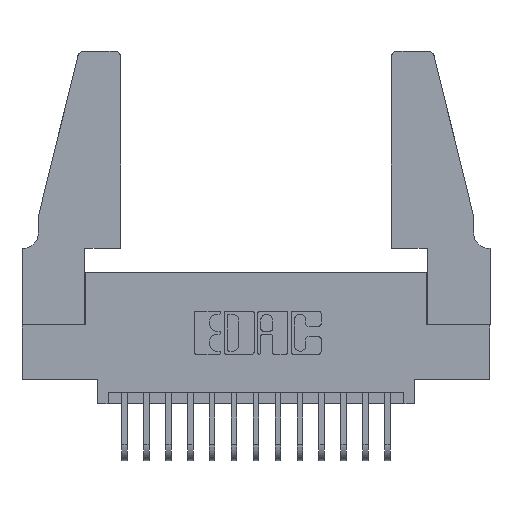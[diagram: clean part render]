
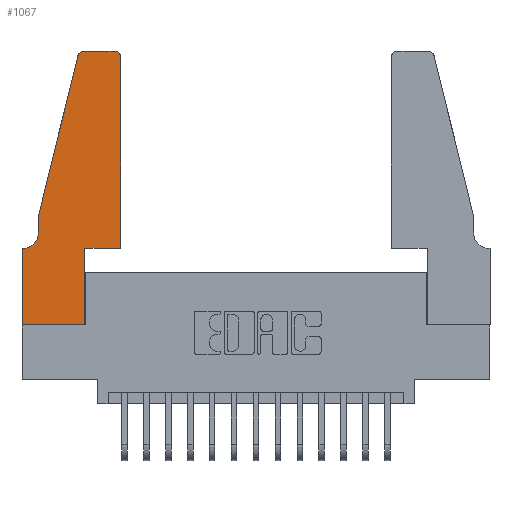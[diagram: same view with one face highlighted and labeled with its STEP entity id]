
A CAD part, top view. The second image highlights one B-rep face of the part: STEP entity #1067.
In plain terms, the highlighted planar face has unit normal (0, 0, 1).
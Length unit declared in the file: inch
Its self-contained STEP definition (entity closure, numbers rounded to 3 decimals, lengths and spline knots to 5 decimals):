
#65 = CARTESIAN_POINT ( 'NONE',  ( 0.0755, 0.42, 0.37 ) ) ;
#125 = EDGE_CURVE ( 'NONE', #2252, #11261, #17638, .T. ) ;
#513 = VERTEX_POINT ( 'NONE', #16929 ) ;
#578 = CARTESIAN_POINT ( 'NONE',  ( 0.4205, 1.25, 0.37 ) ) ;
#634 = AXIS2_PLACEMENT_3D ( 'NONE', #13334, #13268, #6420 ) ;
#637 = CARTESIAN_POINT ( 'NONE',  ( 0.0755, 0.5, 0.37 ) ) ;
#808 = VECTOR ( 'NONE', #11816, 39.37008 ) ;
#824 = LINE ( 'NONE', #6485, #16136 ) ;
#983 = DIRECTION ( 'NONE',  ( -1., 0., 0. ) ) ;
#1049 = FACE_OUTER_BOUND ( 'NONE', #17649, .T. ) ;
#1067 = ADVANCED_FACE ( 'NONE', ( #1049 ), #9913, .T. ) ;
#1149 = VERTEX_POINT ( 'NONE', #11786 ) ;
#1755 = VECTOR ( 'NONE', #6191, 39.37008 ) ;
#1873 = VECTOR ( 'NONE', #3995, 39.37008 ) ;
#1917 = EDGE_CURVE ( 'NONE', #16193, #4725, #12198, .T. ) ;
#2159 = ORIENTED_EDGE ( 'NONE', *, *, #4763, .T. ) ;
#2252 = VERTEX_POINT ( 'NONE', #17783 ) ;
#2263 = VERTEX_POINT ( 'NONE', #15081 ) ;
#2290 = CARTESIAN_POINT ( 'NONE',  ( 0.4505, 0.35, 0.37 ) ) ;
#2453 = VECTOR ( 'NONE', #6379, 39.37008 ) ;
#2570 = EDGE_CURVE ( 'NONE', #1149, #5640, #5826, .T. ) ;
#2689 = DIRECTION ( 'NONE',  ( -1., 0., 0. ) ) ;
#2942 = CARTESIAN_POINT ( 'NONE',  ( 0.4505, 1.22, 0.37 ) ) ;
#3301 = EDGE_CURVE ( 'NONE', #8557, #16193, #14102, .T. ) ;
#3618 = CARTESIAN_POINT ( 'NONE',  ( 0.0055, 0.42, 0.37 ) ) ;
#3658 = LINE ( 'NONE', #13095, #808 ) ;
#3781 = CARTESIAN_POINT ( 'NONE',  ( 0.2605, 1.25, 0.37 ) ) ;
#3995 = DIRECTION ( 'NONE',  ( 0., -1., 0. ) ) ;
#4294 = CARTESIAN_POINT ( 'NONE',  ( 0.4505, 0.35, 0.37 ) ) ;
#4725 = VERTEX_POINT ( 'NONE', #13621 ) ;
#4763 = EDGE_CURVE ( 'NONE', #13131, #1149, #14259, .T. ) ;
#4958 = ORIENTED_EDGE ( 'NONE', *, *, #9117, .T. ) ;
#5321 = AXIS2_PLACEMENT_3D ( 'NONE', #6954, #12606, #12714 ) ;
#5372 = CARTESIAN_POINT ( 'NONE',  ( 0., 0., 0.37 ) ) ;
#5410 = DIRECTION ( 'NONE',  ( 1., 0., 0. ) ) ;
#5640 = VERTEX_POINT ( 'NONE', #15334 ) ;
#5826 = LINE ( 'NONE', #18016, #9329 ) ;
#6191 = DIRECTION ( 'NONE',  ( 1., 0., 0. ) ) ;
#6379 = DIRECTION ( 'NONE',  ( 0., 1., 0. ) ) ;
#6420 = DIRECTION ( 'NONE',  ( 1., 0., 0. ) ) ;
#6443 = EDGE_CURVE ( 'NONE', #4725, #13131, #824, .T. ) ;
#6485 = CARTESIAN_POINT ( 'NONE',  ( 0.0755, 0.35, 0.37 ) ) ;
#6578 = DIRECTION ( 'NONE',  ( -1., 0., 0. ) ) ;
#6681 = EDGE_CURVE ( 'NONE', #2263, #8557, #3658, .T. ) ;
#6808 = LINE ( 'NONE', #3781, #9019 ) ;
#6883 = ORIENTED_EDGE ( 'NONE', *, *, #6443, .T. ) ;
#6954 = CARTESIAN_POINT ( 'NONE',  ( 0., 0.35, 0.37 ) ) ;
#6996 = ORIENTED_EDGE ( 'NONE', *, *, #16022, .T. ) ;
#7057 = AXIS2_PLACEMENT_3D ( 'NONE', #17358, #11962, #12019 ) ;
#7079 = ORIENTED_EDGE ( 'NONE', *, *, #6681, .T. ) ;
#7808 = DIRECTION ( 'NONE',  ( 0., 1., 0. ) ) ;
#7875 = DIRECTION ( 'NONE',  ( 0., 0., -1. ) ) ;
#8315 = ORIENTED_EDGE ( 'NONE', *, *, #10479, .T. ) ;
#8455 = VERTEX_POINT ( 'NONE', #578 ) ;
#8557 = VERTEX_POINT ( 'NONE', #637 ) ;
#9019 = VECTOR ( 'NONE', #983, 39.37008 ) ;
#9117 = EDGE_CURVE ( 'NONE', #513, #2263, #11643, .T. ) ;
#9329 = VECTOR ( 'NONE', #5410, 39.37008 ) ;
#9556 = CARTESIAN_POINT ( 'NONE',  ( 0.0755, 0.5, 0.37 ) ) ;
#9913 = PLANE ( 'NONE',  #5321 ) ;
#10322 = ORIENTED_EDGE ( 'NONE', *, *, #125, .T. ) ;
#10418 = CARTESIAN_POINT ( 'NONE',  ( 0.4505, 0.35, 0.37 ) ) ;
#10479 = EDGE_CURVE ( 'NONE', #8455, #513, #6808, .T. ) ;
#10594 = ORIENTED_EDGE ( 'NONE', *, *, #1917, .T. ) ;
#11016 = EDGE_CURVE ( 'NONE', #5640, #2252, #17238, .T. ) ;
#11101 = AXIS2_PLACEMENT_3D ( 'NONE', #3618, #7875, #6578 ) ;
#11261 = VERTEX_POINT ( 'NONE', #4294 ) ;
#11566 = EDGE_CURVE ( 'NONE', #15791, #8455, #13038, .T. ) ;
#11643 = CIRCLE ( 'NONE', #7057, 0.03 ) ;
#11786 = CARTESIAN_POINT ( 'NONE',  ( 0., 0., 0.37 ) ) ;
#11816 = DIRECTION ( 'NONE',  ( -0.239, -0.971, 0. ) ) ;
#11962 = DIRECTION ( 'NONE',  ( 0., 0., 1. ) ) ;
#12019 = DIRECTION ( 'NONE',  ( 1., 0., 0. ) ) ;
#12107 = VECTOR ( 'NONE', #15157, 39.37008 ) ;
#12198 = CIRCLE ( 'NONE', #11101, 0.07 ) ;
#12606 = DIRECTION ( 'NONE',  ( 0., 0., 1. ) ) ;
#12714 = DIRECTION ( 'NONE',  ( 1., 0., 0. ) ) ;
#13038 = CIRCLE ( 'NONE', #634, 0.03 ) ;
#13090 = LINE ( 'NONE', #2290, #13968 ) ;
#13095 = CARTESIAN_POINT ( 'NONE',  ( 0.0755, 0.5, 0.37 ) ) ;
#13131 = VERTEX_POINT ( 'NONE', #15050 ) ;
#13268 = DIRECTION ( 'NONE',  ( 0., 0., 1. ) ) ;
#13334 = CARTESIAN_POINT ( 'NONE',  ( 0.4205, 1.22, 0.37 ) ) ;
#13358 = CARTESIAN_POINT ( 'NONE',  ( 0.2865, 0.35, 0.37 ) ) ;
#13406 = ORIENTED_EDGE ( 'NONE', *, *, #11016, .T. ) ;
#13621 = CARTESIAN_POINT ( 'NONE',  ( 0.0055, 0.35, 0.37 ) ) ;
#13968 = VECTOR ( 'NONE', #7808, 39.37008 ) ;
#14102 = LINE ( 'NONE', #9556, #1873 ) ;
#14259 = LINE ( 'NONE', #5372, #12107 ) ;
#14768 = ORIENTED_EDGE ( 'NONE', *, *, #11566, .T. ) ;
#15050 = CARTESIAN_POINT ( 'NONE',  ( 0., 0.35, 0.37 ) ) ;
#15081 = CARTESIAN_POINT ( 'NONE',  ( 0.25487, 1.22718, 0.37 ) ) ;
#15157 = DIRECTION ( 'NONE',  ( 0., -1., 0. ) ) ;
#15334 = CARTESIAN_POINT ( 'NONE',  ( 0.2865, 0., 0.37 ) ) ;
#15791 = VERTEX_POINT ( 'NONE', #2942 ) ;
#16022 = EDGE_CURVE ( 'NONE', #11261, #15791, #13090, .T. ) ;
#16093 = ORIENTED_EDGE ( 'NONE', *, *, #3301, .T. ) ;
#16136 = VECTOR ( 'NONE', #2689, 39.37008 ) ;
#16193 = VERTEX_POINT ( 'NONE', #65 ) ;
#16414 = ORIENTED_EDGE ( 'NONE', *, *, #2570, .T. ) ;
#16929 = CARTESIAN_POINT ( 'NONE',  ( 0.284, 1.25, 0.37 ) ) ;
#17238 = LINE ( 'NONE', #13358, #2453 ) ;
#17358 = CARTESIAN_POINT ( 'NONE',  ( 0.284, 1.22, 0.37 ) ) ;
#17638 = LINE ( 'NONE', #10418, #1755 ) ;
#17649 = EDGE_LOOP ( 'NONE', ( #8315, #4958, #7079, #16093, #10594, #6883, #2159, #16414, #13406, #10322, #6996, #14768 ) ) ;
#17783 = CARTESIAN_POINT ( 'NONE',  ( 0.2865, 0.35, 0.37 ) ) ;
#18016 = CARTESIAN_POINT ( 'NONE',  ( 0., 0., 0.37 ) ) ;
